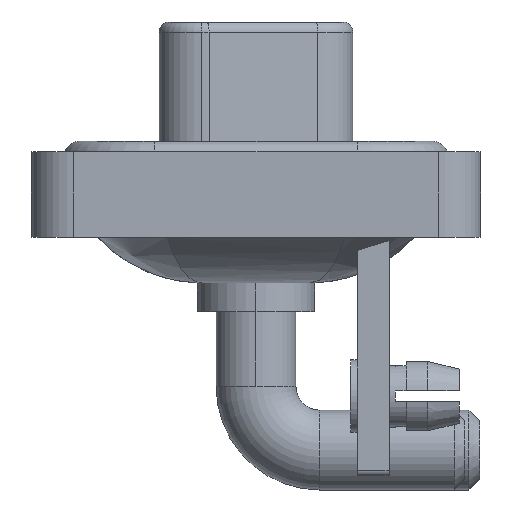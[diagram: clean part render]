
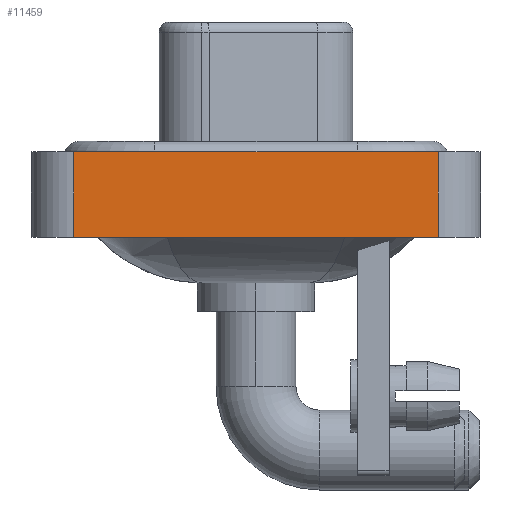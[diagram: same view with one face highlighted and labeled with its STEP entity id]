
A CAD part, left-side view. The second image highlights one B-rep face of the part: STEP entity #11459.
In plain terms, the highlighted planar face has unit normal (-1, 0, 0).
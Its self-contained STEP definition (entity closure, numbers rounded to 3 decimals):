
#45 = AXIS2_PLACEMENT_3D ( 'NONE', #2269, #402, #15628 ) ;
#402 = DIRECTION ( 'NONE',  ( -1., 0., 0. ) ) ;
#734 = PLANE ( 'NONE',  #45 ) ;
#2059 = EDGE_CURVE ( 'NONE', #6338, #11049, #11177, .T. ) ;
#2269 = CARTESIAN_POINT ( 'NONE',  ( -7.3, -8.55, -3.6 ) ) ;
#3369 = EDGE_CURVE ( 'NONE', #14836, #6895, #14153, .T. ) ;
#3699 = VECTOR ( 'NONE', #12928, 1000. ) ;
#3736 = EDGE_LOOP ( 'NONE', ( #5307, #17282, #14908, #16907 ) ) ;
#4030 = CARTESIAN_POINT ( 'NONE',  ( -7.3, -8.55, -3.6 ) ) ;
#4759 = VECTOR ( 'NONE', #17111, 1000. ) ;
#5307 = ORIENTED_EDGE ( 'NONE', *, *, #2059, .T. ) ;
#5821 = EDGE_CURVE ( 'NONE', #6895, #11049, #14366, .T. ) ;
#6338 = VERTEX_POINT ( 'NONE', #4030 ) ;
#6464 = EDGE_CURVE ( 'NONE', #14836, #6338, #13020, .T. ) ;
#6561 = DIRECTION ( 'NONE',  ( 0., -1., 0. ) ) ;
#6895 = VERTEX_POINT ( 'NONE', #19693 ) ;
#8776 = CARTESIAN_POINT ( 'NONE',  ( -7.3, 8.55, -3.6 ) ) ;
#9850 = CARTESIAN_POINT ( 'NONE',  ( -7.3, -8.55, -3.6 ) ) ;
#11049 = VERTEX_POINT ( 'NONE', #13714 ) ;
#11177 = LINE ( 'NONE', #9850, #3699 ) ;
#11459 = ADVANCED_FACE ( 'NONE', ( #11731 ), #734, .T. ) ;
#11731 = FACE_OUTER_BOUND ( 'NONE', #3736, .T. ) ;
#12387 = DIRECTION ( 'NONE',  ( 0., -1., 0. ) ) ;
#12488 = VECTOR ( 'NONE', #12387, 1000. ) ;
#12928 = DIRECTION ( 'NONE',  ( 0., 0., 1. ) ) ;
#13020 = LINE ( 'NONE', #19607, #14466 ) ;
#13714 = CARTESIAN_POINT ( 'NONE',  ( -7.3, -8.55, 0.4 ) ) ;
#14153 = LINE ( 'NONE', #8776, #4759 ) ;
#14366 = LINE ( 'NONE', #20840, #12488 ) ;
#14466 = VECTOR ( 'NONE', #6561, 1000. ) ;
#14836 = VERTEX_POINT ( 'NONE', #15214 ) ;
#14908 = ORIENTED_EDGE ( 'NONE', *, *, #3369, .F. ) ;
#15214 = CARTESIAN_POINT ( 'NONE',  ( -7.3, 8.55, -3.6 ) ) ;
#15628 = DIRECTION ( 'NONE',  ( 0., 0., 1. ) ) ;
#16907 = ORIENTED_EDGE ( 'NONE', *, *, #6464, .T. ) ;
#17111 = DIRECTION ( 'NONE',  ( 0., 0., 1. ) ) ;
#17282 = ORIENTED_EDGE ( 'NONE', *, *, #5821, .F. ) ;
#19607 = CARTESIAN_POINT ( 'NONE',  ( -7.3, -8.55, -3.6 ) ) ;
#19693 = CARTESIAN_POINT ( 'NONE',  ( -7.3, 8.55, 0.4 ) ) ;
#20840 = CARTESIAN_POINT ( 'NONE',  ( -7.3, -8.55, 0.4 ) ) ;
